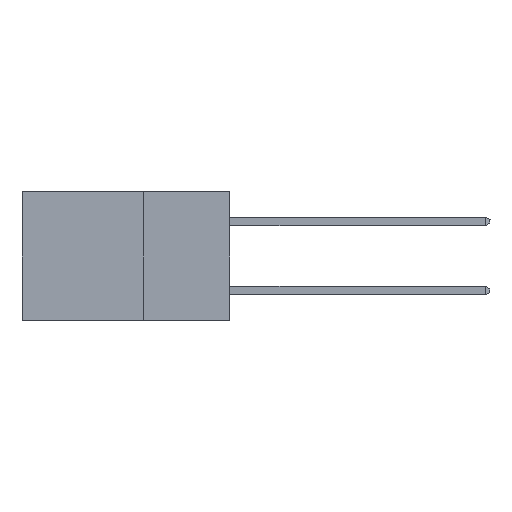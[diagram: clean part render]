
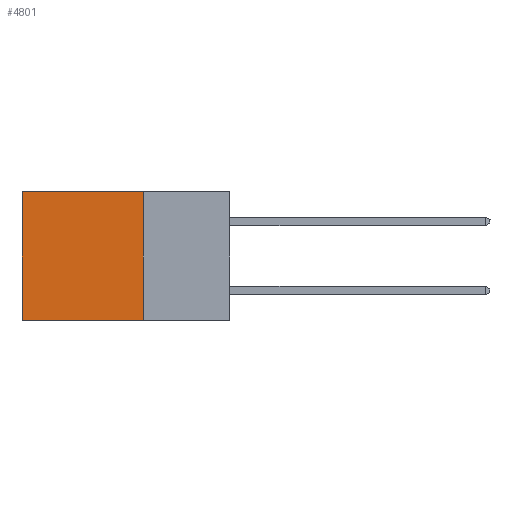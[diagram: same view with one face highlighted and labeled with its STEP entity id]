
A CAD part, left-side view. The second image highlights one B-rep face of the part: STEP entity #4801.
In plain terms, the highlighted planar face has unit normal (-1, 0, 0).
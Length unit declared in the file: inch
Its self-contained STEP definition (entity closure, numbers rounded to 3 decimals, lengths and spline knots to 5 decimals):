
#234 = DIRECTION ( 'NONE',  ( 0., 0., -1. ) ) ;
#373 = VERTEX_POINT ( 'NONE', #7798 ) ;
#1742 = DIRECTION ( 'NONE',  ( 0., 0., -1. ) ) ;
#2179 = CARTESIAN_POINT ( 'NONE',  ( 0.2615, 0.6, -0.37 ) ) ;
#2589 = EDGE_CURVE ( 'NONE', #3596, #11402, #22972, .T. ) ;
#2600 = ORIENTED_EDGE ( 'NONE', *, *, #2589, .F. ) ;
#2959 = FACE_OUTER_BOUND ( 'NONE', #4601, .T. ) ;
#3596 = VERTEX_POINT ( 'NONE', #19518 ) ;
#3683 = LINE ( 'NONE', #21352, #13532 ) ;
#3774 = LINE ( 'NONE', #25451, #11102 ) ;
#4601 = EDGE_LOOP ( 'NONE', ( #23537, #2600, #10227, #25140 ) ) ;
#4801 = ADVANCED_FACE ( 'NONE', ( #2959 ), #24749, .F. ) ;
#4891 = DIRECTION ( 'NONE',  ( 1., 0., 0. ) ) ;
#5142 = DIRECTION ( 'NONE',  ( 0., 0., -1. ) ) ;
#5351 = EDGE_CURVE ( 'NONE', #373, #3596, #3683, .T. ) ;
#6872 = DIRECTION ( 'NONE',  ( 0., 1., 0. ) ) ;
#7028 = EDGE_CURVE ( 'NONE', #373, #11748, #3774, .T. ) ;
#7798 = CARTESIAN_POINT ( 'NONE',  ( 0.2615, 0.25, 0. ) ) ;
#9410 = EDGE_CURVE ( 'NONE', #11748, #11402, #13654, .T. ) ;
#10227 = ORIENTED_EDGE ( 'NONE', *, *, #5351, .F. ) ;
#10732 = VECTOR ( 'NONE', #234, 39.37008 ) ;
#11102 = VECTOR ( 'NONE', #11266, 39.37008 ) ;
#11266 = DIRECTION ( 'NONE',  ( 0., 1., 0. ) ) ;
#11402 = VERTEX_POINT ( 'NONE', #22817 ) ;
#11748 = VERTEX_POINT ( 'NONE', #14173 ) ;
#13532 = VECTOR ( 'NONE', #1742, 39.37008 ) ;
#13654 = LINE ( 'NONE', #2179, #10732 ) ;
#14173 = CARTESIAN_POINT ( 'NONE',  ( 0.2615, 0.6, 0. ) ) ;
#16804 = AXIS2_PLACEMENT_3D ( 'NONE', #21121, #4891, #5142 ) ;
#17158 = CARTESIAN_POINT ( 'NONE',  ( 0.2615, 0.25, -0.37 ) ) ;
#19518 = CARTESIAN_POINT ( 'NONE',  ( 0.2615, 0.25, -0.37 ) ) ;
#21121 = CARTESIAN_POINT ( 'NONE',  ( 0.2615, 0.25, -0.37 ) ) ;
#21352 = CARTESIAN_POINT ( 'NONE',  ( 0.2615, 0.25, -0.37 ) ) ;
#22817 = CARTESIAN_POINT ( 'NONE',  ( 0.2615, 0.6, -0.37 ) ) ;
#22972 = LINE ( 'NONE', #17158, #23842 ) ;
#23537 = ORIENTED_EDGE ( 'NONE', *, *, #9410, .T. ) ;
#23842 = VECTOR ( 'NONE', #6872, 39.37008 ) ;
#24749 = PLANE ( 'NONE',  #16804 ) ;
#25140 = ORIENTED_EDGE ( 'NONE', *, *, #7028, .T. ) ;
#25451 = CARTESIAN_POINT ( 'NONE',  ( 0.2615, 0.25, 0. ) ) ;
